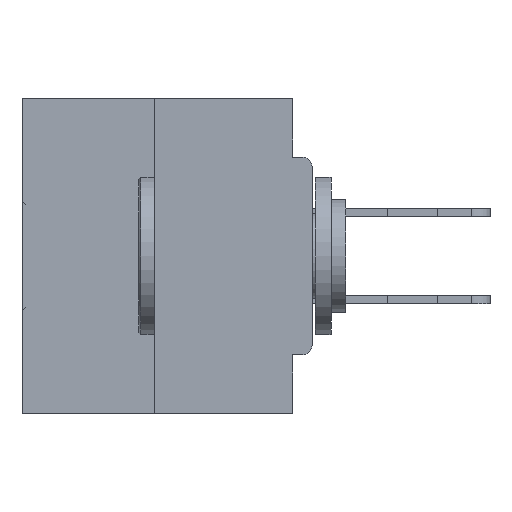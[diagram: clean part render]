
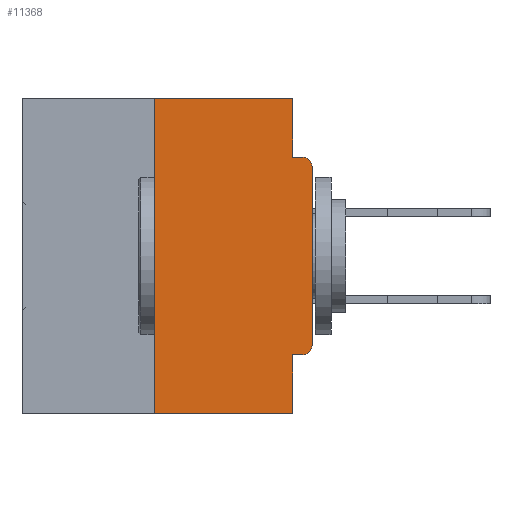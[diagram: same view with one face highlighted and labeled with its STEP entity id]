
A CAD part, left-side view. The second image highlights one B-rep face of the part: STEP entity #11368.
In plain terms, the highlighted planar face has unit normal (-1, 0, 0).
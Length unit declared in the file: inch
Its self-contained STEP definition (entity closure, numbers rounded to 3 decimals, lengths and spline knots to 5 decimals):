
#222 = DIRECTION ( 'NONE',  ( 0., 1., 0. ) ) ;
#562 = CARTESIAN_POINT ( 'NONE',  ( 0., 0.015, -0.0935 ) ) ;
#1131 = EDGE_CURVE ( 'NONE', #34065, #17571, #26425, .T. ) ;
#2666 = VECTOR ( 'NONE', #3309, 39.37008 ) ;
#2816 = VECTOR ( 'NONE', #222, 39.37008 ) ;
#3060 = CARTESIAN_POINT ( 'NONE',  ( 0., 0.46, 0. ) ) ;
#3309 = DIRECTION ( 'NONE',  ( 0., -1., 0. ) ) ;
#5048 = EDGE_CURVE ( 'NONE', #39881, #19835, #20811, .T. ) ;
#5153 = VERTEX_POINT ( 'NONE', #9043 ) ;
#5426 = CARTESIAN_POINT ( 'NONE',  ( 0., 0., -0.3915 ) ) ;
#5701 = LINE ( 'NONE', #8136, #23916 ) ;
#6063 = ORIENTED_EDGE ( 'NONE', *, *, #34529, .F. ) ;
#6733 = EDGE_CURVE ( 'NONE', #33172, #24492, #21284, .T. ) ;
#7993 = ORIENTED_EDGE ( 'NONE', *, *, #6733, .F. ) ;
#8136 = CARTESIAN_POINT ( 'NONE',  ( 0., 0.46, -0.5 ) ) ;
#9043 = CARTESIAN_POINT ( 'NONE',  ( 0., 0.25, -0.5 ) ) ;
#10510 = CARTESIAN_POINT ( 'NONE',  ( 0., 0.015, -0.4065 ) ) ;
#10577 = CARTESIAN_POINT ( 'NONE',  ( 0., 0.46, 0. ) ) ;
#11090 = EDGE_CURVE ( 'NONE', #28120, #33172, #17014, .T. ) ;
#11368 = ADVANCED_FACE ( 'NONE', ( #31304 ), #20607, .F. ) ;
#13031 = DIRECTION ( 'NONE',  ( 0., 0., 1. ) ) ;
#13152 = CARTESIAN_POINT ( 'NONE',  ( 0., 0.25, 0. ) ) ;
#13710 = VECTOR ( 'NONE', #21815, 39.37008 ) ;
#14253 = ORIENTED_EDGE ( 'NONE', *, *, #42191, .F. ) ;
#14313 = DIRECTION ( 'NONE',  ( 0., 0., -1. ) ) ;
#14617 = DIRECTION ( 'NONE',  ( 0., -1., 0. ) ) ;
#15080 = CARTESIAN_POINT ( 'NONE',  ( 0., 0.031, -0.4065 ) ) ;
#15142 = CARTESIAN_POINT ( 'NONE',  ( 0., 0.25, 0. ) ) ;
#15735 = DIRECTION ( 'NONE',  ( -1., 0., 0. ) ) ;
#16072 = CARTESIAN_POINT ( 'NONE',  ( 0., 0., -0.1085 ) ) ;
#16223 = CARTESIAN_POINT ( 'NONE',  ( 0., 0.031, 0. ) ) ;
#17014 = LINE ( 'NONE', #10577, #13710 ) ;
#17571 = VERTEX_POINT ( 'NONE', #15080 ) ;
#18732 = VECTOR ( 'NONE', #40917, 39.37008 ) ;
#19445 = AXIS2_PLACEMENT_3D ( 'NONE', #36319, #29571, #29411 ) ;
#19690 = CARTESIAN_POINT ( 'NONE',  ( 0., 0.031, -0.5 ) ) ;
#19835 = VERTEX_POINT ( 'NONE', #562 ) ;
#20607 = PLANE ( 'NONE',  #26447 ) ;
#20811 = CIRCLE ( 'NONE', #38067, 0.015 ) ;
#21284 = LINE ( 'NONE', #29075, #25640 ) ;
#21815 = DIRECTION ( 'NONE',  ( 0., -1., 0. ) ) ;
#22284 = CIRCLE ( 'NONE', #19445, 0.015 ) ;
#22502 = VECTOR ( 'NONE', #13031, 39.37008 ) ;
#23091 = ORIENTED_EDGE ( 'NONE', *, *, #36931, .T. ) ;
#23916 = VECTOR ( 'NONE', #14617, 39.37008 ) ;
#24151 = CARTESIAN_POINT ( 'NONE',  ( 0., 0., 0. ) ) ;
#24492 = VERTEX_POINT ( 'NONE', #37133 ) ;
#25199 = DIRECTION ( 'NONE',  ( 1., 0., 0. ) ) ;
#25520 = EDGE_CURVE ( 'NONE', #5153, #33529, #5701, .T. ) ;
#25640 = VECTOR ( 'NONE', #32595, 39.37008 ) ;
#26203 = ORIENTED_EDGE ( 'NONE', *, *, #44570, .T. ) ;
#26425 = LINE ( 'NONE', #35389, #2816 ) ;
#26447 = AXIS2_PLACEMENT_3D ( 'NONE', #3060, #25199, #14313 ) ;
#27989 = LINE ( 'NONE', #19690, #18732 ) ;
#28120 = VERTEX_POINT ( 'NONE', #13152 ) ;
#29075 = CARTESIAN_POINT ( 'NONE',  ( 0., 0.031, 0. ) ) ;
#29411 = DIRECTION ( 'NONE',  ( 0., 0., -1. ) ) ;
#29571 = DIRECTION ( 'NONE',  ( -1., 0., 0. ) ) ;
#30042 = VECTOR ( 'NONE', #41830, 39.37008 ) ;
#30709 = VERTEX_POINT ( 'NONE', #5426 ) ;
#31304 = FACE_OUTER_BOUND ( 'NONE', #37696, .T. ) ;
#31461 = CARTESIAN_POINT ( 'NONE',  ( 0., 0., -0.0935 ) ) ;
#31908 = CARTESIAN_POINT ( 'NONE',  ( 0., 0.031, -0.5 ) ) ;
#32595 = DIRECTION ( 'NONE',  ( 0., 0., -1. ) ) ;
#32960 = ORIENTED_EDGE ( 'NONE', *, *, #25520, .T. ) ;
#33093 = ORIENTED_EDGE ( 'NONE', *, *, #11090, .F. ) ;
#33172 = VERTEX_POINT ( 'NONE', #16223 ) ;
#33225 = CARTESIAN_POINT ( 'NONE',  ( 0., 0.015, -0.1085 ) ) ;
#33529 = VERTEX_POINT ( 'NONE', #31908 ) ;
#34065 = VERTEX_POINT ( 'NONE', #10510 ) ;
#34529 = EDGE_CURVE ( 'NONE', #17571, #33529, #27989, .T. ) ;
#34999 = EDGE_CURVE ( 'NONE', #24492, #19835, #43958, .T. ) ;
#35389 = CARTESIAN_POINT ( 'NONE',  ( 0., 0., -0.4065 ) ) ;
#36319 = CARTESIAN_POINT ( 'NONE',  ( 0., 0.015, -0.3915 ) ) ;
#36931 = EDGE_CURVE ( 'NONE', #34065, #30709, #22284, .T. ) ;
#37133 = CARTESIAN_POINT ( 'NONE',  ( 0., 0.031, -0.0935 ) ) ;
#37696 = EDGE_LOOP ( 'NONE', ( #33093, #14253, #32960, #6063, #41111, #23091, #26203, #41330, #45066, #7993 ) ) ;
#38067 = AXIS2_PLACEMENT_3D ( 'NONE', #33225, #15735, #40339 ) ;
#39424 = LINE ( 'NONE', #24151, #30042 ) ;
#39598 = LINE ( 'NONE', #15142, #22502 ) ;
#39881 = VERTEX_POINT ( 'NONE', #16072 ) ;
#40339 = DIRECTION ( 'NONE',  ( 0., 0., -1. ) ) ;
#40917 = DIRECTION ( 'NONE',  ( 0., 0., -1. ) ) ;
#41111 = ORIENTED_EDGE ( 'NONE', *, *, #1131, .F. ) ;
#41330 = ORIENTED_EDGE ( 'NONE', *, *, #5048, .T. ) ;
#41830 = DIRECTION ( 'NONE',  ( 0., 0., 1. ) ) ;
#42191 = EDGE_CURVE ( 'NONE', #5153, #28120, #39598, .T. ) ;
#43958 = LINE ( 'NONE', #31461, #2666 ) ;
#44570 = EDGE_CURVE ( 'NONE', #30709, #39881, #39424, .T. ) ;
#45066 = ORIENTED_EDGE ( 'NONE', *, *, #34999, .F. ) ;
